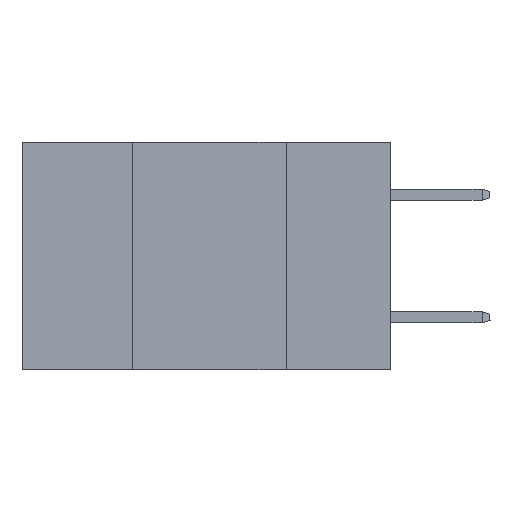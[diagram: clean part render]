
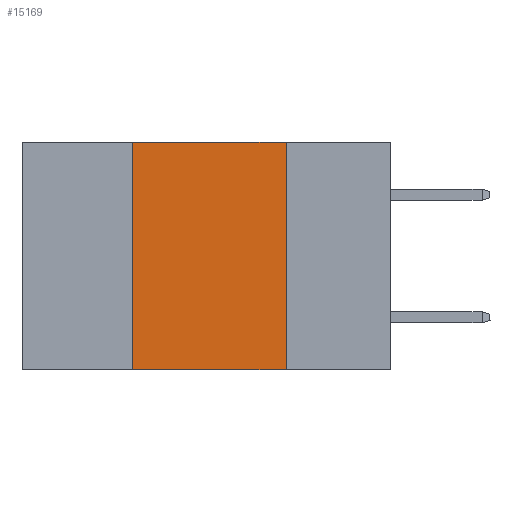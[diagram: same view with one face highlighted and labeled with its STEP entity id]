
A CAD part, left-side view. The second image highlights one B-rep face of the part: STEP entity #15169.
In plain terms, the highlighted planar face has unit normal (-1, 0, 0).
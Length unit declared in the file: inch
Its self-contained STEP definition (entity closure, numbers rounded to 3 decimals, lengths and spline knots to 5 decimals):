
#53 = CARTESIAN_POINT ( 'NONE',  ( 0., 0.17, 0. ) ) ;
#844 = LINE ( 'NONE', #4330, #14350 ) ;
#1804 = CARTESIAN_POINT ( 'NONE',  ( 0., 0.42, 0. ) ) ;
#1828 = EDGE_LOOP ( 'NONE', ( #6203, #3625, #13547, #8020 ) ) ;
#2708 = DIRECTION ( 'NONE',  ( 1., 0., 0. ) ) ;
#3625 = ORIENTED_EDGE ( 'NONE', *, *, #5683, .F. ) ;
#4321 = LINE ( 'NONE', #14917, #17677 ) ;
#4330 = CARTESIAN_POINT ( 'NONE',  ( 0., 0.6, 0. ) ) ;
#4672 = LINE ( 'NONE', #16906, #17992 ) ;
#5467 = VECTOR ( 'NONE', #21864, 39.37008 ) ;
#5683 = EDGE_CURVE ( 'NONE', #10487, #14849, #844, .T. ) ;
#6203 = ORIENTED_EDGE ( 'NONE', *, *, #11314, .F. ) ;
#6272 = CARTESIAN_POINT ( 'NONE',  ( 0., 0.17, -0.37 ) ) ;
#7739 = EDGE_CURVE ( 'NONE', #11243, #13860, #4672, .T. ) ;
#8020 = ORIENTED_EDGE ( 'NONE', *, *, #7739, .T. ) ;
#8922 = EDGE_CURVE ( 'NONE', #11243, #10487, #4321, .T. ) ;
#9781 = CARTESIAN_POINT ( 'NONE',  ( 0., 0.6, 0. ) ) ;
#10487 = VERTEX_POINT ( 'NONE', #1804 ) ;
#10592 = AXIS2_PLACEMENT_3D ( 'NONE', #9781, #2708, #14951 ) ;
#11243 = VERTEX_POINT ( 'NONE', #19991 ) ;
#11314 = EDGE_CURVE ( 'NONE', #14849, #13860, #19810, .T. ) ;
#13547 = ORIENTED_EDGE ( 'NONE', *, *, #8922, .F. ) ;
#13860 = VERTEX_POINT ( 'NONE', #6272 ) ;
#14350 = VECTOR ( 'NONE', #14816, 39.37008 ) ;
#14816 = DIRECTION ( 'NONE',  ( 0., -1., 0. ) ) ;
#14849 = VERTEX_POINT ( 'NONE', #53 ) ;
#14874 = PLANE ( 'NONE',  #10592 ) ;
#14917 = CARTESIAN_POINT ( 'NONE',  ( 0., 0.42, 0. ) ) ;
#14951 = DIRECTION ( 'NONE',  ( 0., 0., -1. ) ) ;
#15169 = ADVANCED_FACE ( 'NONE', ( #21027 ), #14874, .F. ) ;
#16636 = DIRECTION ( 'NONE',  ( 0., 0., 1. ) ) ;
#16906 = CARTESIAN_POINT ( 'NONE',  ( 0., 0.6, -0.37 ) ) ;
#17677 = VECTOR ( 'NONE', #16636, 39.37008 ) ;
#17992 = VECTOR ( 'NONE', #22082, 39.37008 ) ;
#18398 = CARTESIAN_POINT ( 'NONE',  ( 0., 0.17, 0. ) ) ;
#19810 = LINE ( 'NONE', #18398, #5467 ) ;
#19991 = CARTESIAN_POINT ( 'NONE',  ( 0., 0.42, -0.37 ) ) ;
#21027 = FACE_OUTER_BOUND ( 'NONE', #1828, .T. ) ;
#21864 = DIRECTION ( 'NONE',  ( 0., 0., -1. ) ) ;
#22082 = DIRECTION ( 'NONE',  ( 0., -1., 0. ) ) ;
